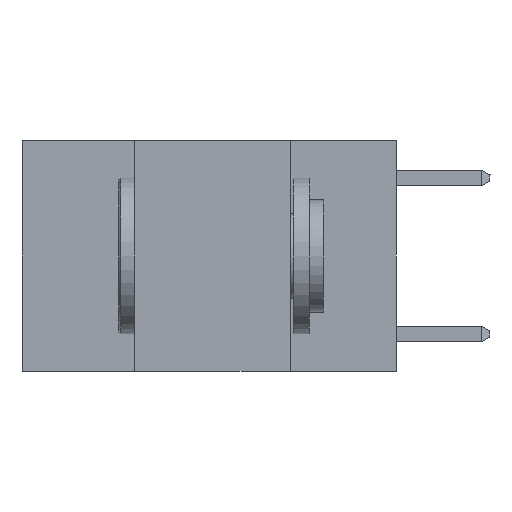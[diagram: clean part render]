
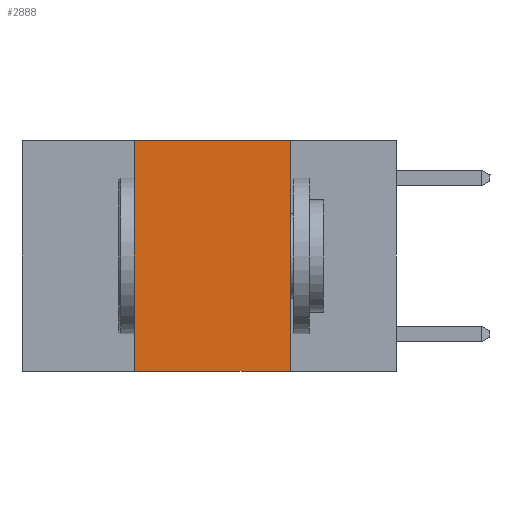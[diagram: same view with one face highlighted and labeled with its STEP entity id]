
A CAD part, left-side view. The second image highlights one B-rep face of the part: STEP entity #2888.
In plain terms, the highlighted planar face has unit normal (-1, 0, 0).
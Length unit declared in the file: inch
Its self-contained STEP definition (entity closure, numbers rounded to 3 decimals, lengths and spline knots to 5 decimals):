
#19 = VERTEX_POINT ( 'NONE', #1667 ) ;
#116 = DIRECTION ( 'NONE',  ( 0., -1., 0. ) ) ;
#214 = DIRECTION ( 'NONE',  ( 0., 0., 1. ) ) ;
#646 = LINE ( 'NONE', #3591, #7286 ) ;
#909 = DIRECTION ( 'NONE',  ( 0., 0., -1. ) ) ;
#1667 = CARTESIAN_POINT ( 'NONE',  ( 0., 0.17, -0.37 ) ) ;
#1876 = VERTEX_POINT ( 'NONE', #9156 ) ;
#2149 = ORIENTED_EDGE ( 'NONE', *, *, #6329, .F. ) ;
#2288 = DIRECTION ( 'NONE',  ( 0., 0., -1. ) ) ;
#2470 = EDGE_CURVE ( 'NONE', #9170, #19, #646, .T. ) ;
#2513 = ORIENTED_EDGE ( 'NONE', *, *, #9077, .F. ) ;
#2707 = LINE ( 'NONE', #6222, #5525 ) ;
#2888 = ADVANCED_FACE ( 'NONE', ( #6636 ), #3801, .F. ) ;
#3293 = EDGE_CURVE ( 'NONE', #4360, #19, #8143, .T. ) ;
#3591 = CARTESIAN_POINT ( 'NONE',  ( 0., 0.6, -0.37 ) ) ;
#3801 = PLANE ( 'NONE',  #9286 ) ;
#4360 = VERTEX_POINT ( 'NONE', #7480 ) ;
#4507 = CARTESIAN_POINT ( 'NONE',  ( 0., 0.17, 0. ) ) ;
#4569 = DIRECTION ( 'NONE',  ( 1., 0., 0. ) ) ;
#5525 = VECTOR ( 'NONE', #9144, 39.37008 ) ;
#5952 = CARTESIAN_POINT ( 'NONE',  ( 0., 0.6, 0. ) ) ;
#6162 = CARTESIAN_POINT ( 'NONE',  ( 0., 0.42, -0.37 ) ) ;
#6215 = ORIENTED_EDGE ( 'NONE', *, *, #3293, .F. ) ;
#6222 = CARTESIAN_POINT ( 'NONE',  ( 0., 0.6, 0. ) ) ;
#6245 = VECTOR ( 'NONE', #2288, 39.37008 ) ;
#6329 = EDGE_CURVE ( 'NONE', #1876, #4360, #2707, .T. ) ;
#6609 = VECTOR ( 'NONE', #214, 39.37008 ) ;
#6636 = FACE_OUTER_BOUND ( 'NONE', #7826, .T. ) ;
#7286 = VECTOR ( 'NONE', #116, 39.37008 ) ;
#7472 = ORIENTED_EDGE ( 'NONE', *, *, #2470, .T. ) ;
#7480 = CARTESIAN_POINT ( 'NONE',  ( 0., 0.17, 0. ) ) ;
#7826 = EDGE_LOOP ( 'NONE', ( #6215, #2149, #2513, #7472 ) ) ;
#8143 = LINE ( 'NONE', #4507, #6245 ) ;
#8331 = LINE ( 'NONE', #8900, #6609 ) ;
#8900 = CARTESIAN_POINT ( 'NONE',  ( 0., 0.42, 0. ) ) ;
#9077 = EDGE_CURVE ( 'NONE', #9170, #1876, #8331, .T. ) ;
#9144 = DIRECTION ( 'NONE',  ( 0., -1., 0. ) ) ;
#9156 = CARTESIAN_POINT ( 'NONE',  ( 0., 0.42, 0. ) ) ;
#9170 = VERTEX_POINT ( 'NONE', #6162 ) ;
#9286 = AXIS2_PLACEMENT_3D ( 'NONE', #5952, #4569, #909 ) ;
